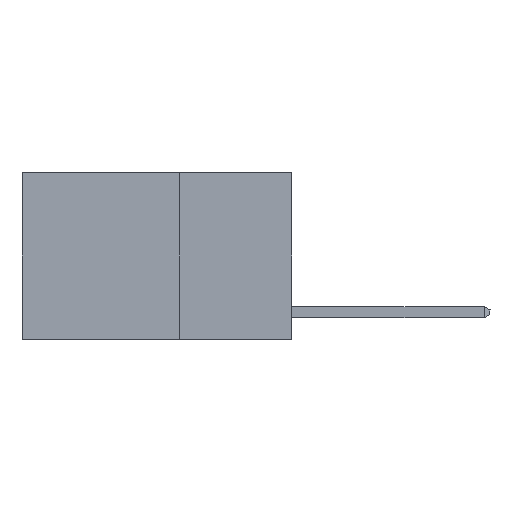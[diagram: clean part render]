
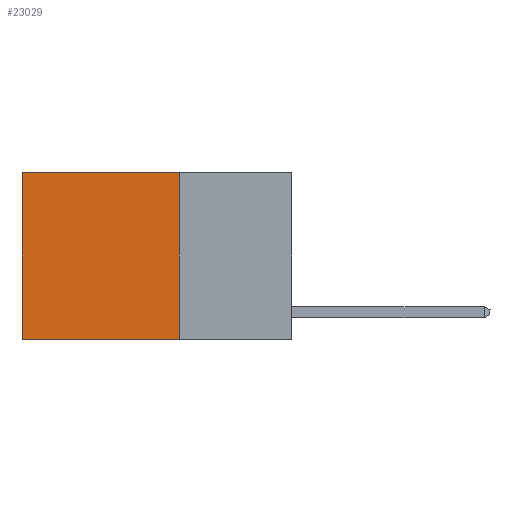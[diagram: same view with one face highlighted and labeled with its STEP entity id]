
A CAD part, left-side view. The second image highlights one B-rep face of the part: STEP entity #23029.
In plain terms, the highlighted planar face has unit normal (-1, 0, 0).
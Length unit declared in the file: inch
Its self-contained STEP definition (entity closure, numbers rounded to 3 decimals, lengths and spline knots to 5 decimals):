
#1324 = EDGE_CURVE ( 'NONE', #18385, #14157, #5247, .T. ) ;
#2828 = DIRECTION ( 'NONE',  ( 1., 0., 0. ) ) ;
#4085 = VECTOR ( 'NONE', #22370, 39.37008 ) ;
#4125 = VERTEX_POINT ( 'NONE', #19317 ) ;
#4293 = ORIENTED_EDGE ( 'NONE', *, *, #19311, .T. ) ;
#4570 = FACE_OUTER_BOUND ( 'NONE', #6725, .T. ) ;
#5247 = LINE ( 'NONE', #17130, #18694 ) ;
#6725 = EDGE_LOOP ( 'NONE', ( #4293, #22633, #9635, #19297 ) ) ;
#7019 = CARTESIAN_POINT ( 'NONE',  ( 0.2625, 0.6, 0. ) ) ;
#7103 = VECTOR ( 'NONE', #19661, 39.37008 ) ;
#7666 = LINE ( 'NONE', #7019, #16769 ) ;
#8276 = LINE ( 'NONE', #8759, #7103 ) ;
#8759 = CARTESIAN_POINT ( 'NONE',  ( 0.2625, 0.25, 0. ) ) ;
#9635 = ORIENTED_EDGE ( 'NONE', *, *, #18298, .F. ) ;
#10723 = DIRECTION ( 'NONE',  ( 0., 0., -1. ) ) ;
#10922 = CARTESIAN_POINT ( 'NONE',  ( 0.2625, 0.6, -0.37 ) ) ;
#12063 = AXIS2_PLACEMENT_3D ( 'NONE', #13895, #2828, #15727 ) ;
#13466 = CARTESIAN_POINT ( 'NONE',  ( 0.2625, 0.25, -0.37 ) ) ;
#13895 = CARTESIAN_POINT ( 'NONE',  ( 0.2625, 0.25, 0. ) ) ;
#14157 = VERTEX_POINT ( 'NONE', #10922 ) ;
#15342 = VERTEX_POINT ( 'NONE', #23677 ) ;
#15727 = DIRECTION ( 'NONE',  ( 0., 0., -1. ) ) ;
#16508 = EDGE_CURVE ( 'NONE', #4125, #15342, #8276, .T. ) ;
#16769 = VECTOR ( 'NONE', #10723, 39.37008 ) ;
#17130 = CARTESIAN_POINT ( 'NONE',  ( 0.2625, 0.25, -0.37 ) ) ;
#18298 = EDGE_CURVE ( 'NONE', #4125, #18385, #18702, .T. ) ;
#18385 = VERTEX_POINT ( 'NONE', #13466 ) ;
#18694 = VECTOR ( 'NONE', #20719, 39.37008 ) ;
#18702 = LINE ( 'NONE', #20530, #4085 ) ;
#19297 = ORIENTED_EDGE ( 'NONE', *, *, #16508, .T. ) ;
#19311 = EDGE_CURVE ( 'NONE', #15342, #14157, #7666, .T. ) ;
#19317 = CARTESIAN_POINT ( 'NONE',  ( 0.2625, 0.25, 0. ) ) ;
#19661 = DIRECTION ( 'NONE',  ( 0., 1., 0. ) ) ;
#20530 = CARTESIAN_POINT ( 'NONE',  ( 0.2625, 0.25, 0. ) ) ;
#20719 = DIRECTION ( 'NONE',  ( 0., 1., 0. ) ) ;
#21126 = PLANE ( 'NONE',  #12063 ) ;
#22370 = DIRECTION ( 'NONE',  ( 0., 0., -1. ) ) ;
#22633 = ORIENTED_EDGE ( 'NONE', *, *, #1324, .F. ) ;
#23029 = ADVANCED_FACE ( 'NONE', ( #4570 ), #21126, .F. ) ;
#23677 = CARTESIAN_POINT ( 'NONE',  ( 0.2625, 0.6, 0. ) ) ;
